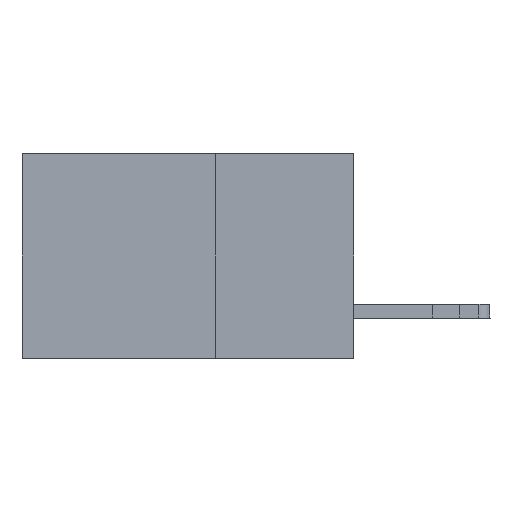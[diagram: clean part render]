
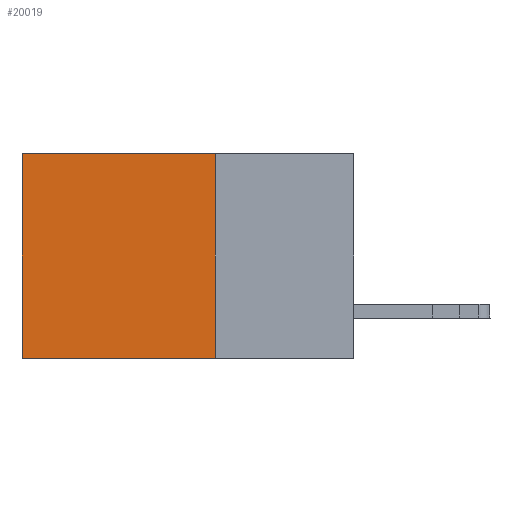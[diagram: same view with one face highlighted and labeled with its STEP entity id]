
A CAD part, left-side view. The second image highlights one B-rep face of the part: STEP entity #20019.
In plain terms, the highlighted planar face has unit normal (-1, 0, 0).
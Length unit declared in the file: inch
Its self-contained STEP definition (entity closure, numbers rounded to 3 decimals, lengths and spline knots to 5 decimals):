
#546 = VECTOR ( 'NONE', #6658, 39.37008 ) ;
#886 = LINE ( 'NONE', #24730, #546 ) ;
#2560 = DIRECTION ( 'NONE',  ( 0., 1., 0. ) ) ;
#2667 = AXIS2_PLACEMENT_3D ( 'NONE', #22478, #2859, #7277 ) ;
#2859 = DIRECTION ( 'NONE',  ( 1., 0., 0. ) ) ;
#3351 = CARTESIAN_POINT ( 'NONE',  ( 0.2875, 0.25, 0. ) ) ;
#4073 = VECTOR ( 'NONE', #2560, 39.37008 ) ;
#5620 = VERTEX_POINT ( 'NONE', #10972 ) ;
#6658 = DIRECTION ( 'NONE',  ( 0., 1., 0. ) ) ;
#7277 = DIRECTION ( 'NONE',  ( 0., 0., -1. ) ) ;
#7363 = PLANE ( 'NONE',  #2667 ) ;
#7469 = DIRECTION ( 'NONE',  ( 0., 0., -1. ) ) ;
#9170 = EDGE_CURVE ( 'NONE', #23751, #5620, #22284, .T. ) ;
#9578 = DIRECTION ( 'NONE',  ( 0., 0., -1. ) ) ;
#10142 = LINE ( 'NONE', #22758, #25614 ) ;
#10354 = FACE_OUTER_BOUND ( 'NONE', #20057, .T. ) ;
#10580 = EDGE_CURVE ( 'NONE', #19565, #11196, #886, .T. ) ;
#10972 = CARTESIAN_POINT ( 'NONE',  ( 0.2875, 0.6, 0. ) ) ;
#11196 = VERTEX_POINT ( 'NONE', #13926 ) ;
#11211 = EDGE_CURVE ( 'NONE', #5620, #11196, #22745, .T. ) ;
#12182 = ORIENTED_EDGE ( 'NONE', *, *, #24669, .F. ) ;
#13926 = CARTESIAN_POINT ( 'NONE',  ( 0.2875, 0.6, -0.37 ) ) ;
#17318 = ORIENTED_EDGE ( 'NONE', *, *, #11211, .T. ) ;
#19103 = ORIENTED_EDGE ( 'NONE', *, *, #9170, .T. ) ;
#19565 = VERTEX_POINT ( 'NONE', #23841 ) ;
#19662 = CARTESIAN_POINT ( 'NONE',  ( 0.2875, 0.25, 0. ) ) ;
#20019 = ADVANCED_FACE ( 'NONE', ( #10354 ), #7363, .F. ) ;
#20057 = EDGE_LOOP ( 'NONE', ( #17318, #21762, #12182, #19103 ) ) ;
#21762 = ORIENTED_EDGE ( 'NONE', *, *, #10580, .F. ) ;
#22284 = LINE ( 'NONE', #19662, #4073 ) ;
#22478 = CARTESIAN_POINT ( 'NONE',  ( 0.2875, 0.25, 0. ) ) ;
#22745 = LINE ( 'NONE', #26988, #27521 ) ;
#22758 = CARTESIAN_POINT ( 'NONE',  ( 0.2875, 0.25, 0. ) ) ;
#23751 = VERTEX_POINT ( 'NONE', #3351 ) ;
#23841 = CARTESIAN_POINT ( 'NONE',  ( 0.2875, 0.25, -0.37 ) ) ;
#24669 = EDGE_CURVE ( 'NONE', #23751, #19565, #10142, .T. ) ;
#24730 = CARTESIAN_POINT ( 'NONE',  ( 0.2875, 0.25, -0.37 ) ) ;
#25614 = VECTOR ( 'NONE', #9578, 39.37008 ) ;
#26988 = CARTESIAN_POINT ( 'NONE',  ( 0.2875, 0.6, 0. ) ) ;
#27521 = VECTOR ( 'NONE', #7469, 39.37008 ) ;
